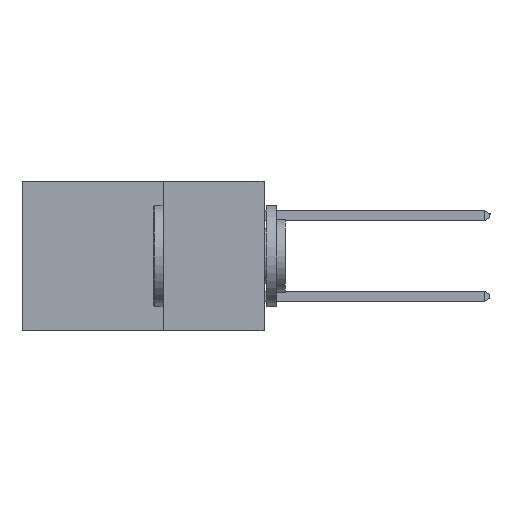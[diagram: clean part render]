
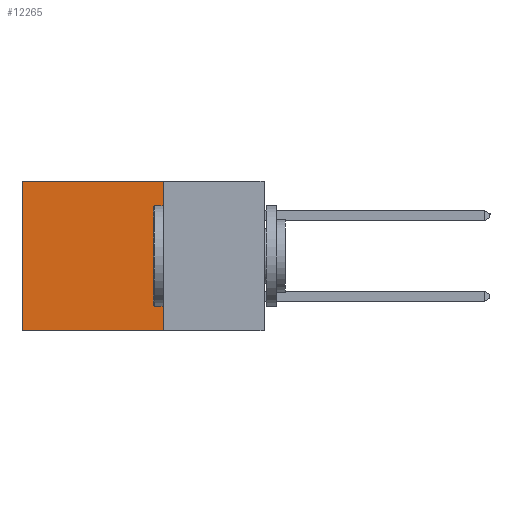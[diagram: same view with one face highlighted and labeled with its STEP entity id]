
A CAD part, left-side view. The second image highlights one B-rep face of the part: STEP entity #12265.
In plain terms, the highlighted planar face has unit normal (-1, 0, 0).
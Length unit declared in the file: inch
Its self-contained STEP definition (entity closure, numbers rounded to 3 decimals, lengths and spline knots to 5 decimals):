
#662 = DIRECTION ( 'NONE',  ( 1., 0., 0. ) ) ;
#748 = EDGE_CURVE ( 'NONE', #22641, #20299, #19825, .T. ) ;
#1297 = DIRECTION ( 'NONE',  ( 0., 1., 0. ) ) ;
#1557 = CARTESIAN_POINT ( 'NONE',  ( 0.2615, 0.25, 0. ) ) ;
#1861 = CARTESIAN_POINT ( 'NONE',  ( 0.2615, 0.25, -0.37 ) ) ;
#2840 = AXIS2_PLACEMENT_3D ( 'NONE', #23645, #662, #15559 ) ;
#3161 = VECTOR ( 'NONE', #1297, 39.37008 ) ;
#3678 = CARTESIAN_POINT ( 'NONE',  ( 0.2615, 0.25, -0.37 ) ) ;
#4022 = LINE ( 'NONE', #1861, #17274 ) ;
#4068 = VECTOR ( 'NONE', #26313, 39.37008 ) ;
#4404 = EDGE_LOOP ( 'NONE', ( #23438, #19910, #12541, #13023 ) ) ;
#4945 = LINE ( 'NONE', #16974, #21809 ) ;
#7323 = FACE_OUTER_BOUND ( 'NONE', #4404, .T. ) ;
#8329 = VERTEX_POINT ( 'NONE', #3678 ) ;
#10783 = CARTESIAN_POINT ( 'NONE',  ( 0.2615, 0.6, -0.37 ) ) ;
#12265 = ADVANCED_FACE ( 'NONE', ( #7323 ), #15156, .F. ) ;
#12541 = ORIENTED_EDGE ( 'NONE', *, *, #22267, .F. ) ;
#12747 = VERTEX_POINT ( 'NONE', #10783 ) ;
#13023 = ORIENTED_EDGE ( 'NONE', *, *, #748, .T. ) ;
#13257 = EDGE_CURVE ( 'NONE', #20299, #12747, #4945, .T. ) ;
#14011 = CARTESIAN_POINT ( 'NONE',  ( 0.2615, 0.25, -0.37 ) ) ;
#15156 = PLANE ( 'NONE',  #2840 ) ;
#15358 = DIRECTION ( 'NONE',  ( 0., 0., -1. ) ) ;
#15559 = DIRECTION ( 'NONE',  ( 0., 0., -1. ) ) ;
#16974 = CARTESIAN_POINT ( 'NONE',  ( 0.2615, 0.6, -0.37 ) ) ;
#17274 = VECTOR ( 'NONE', #24571, 39.37008 ) ;
#18073 = LINE ( 'NONE', #14011, #4068 ) ;
#18370 = CARTESIAN_POINT ( 'NONE',  ( 0.2615, 0.6, 0. ) ) ;
#18880 = EDGE_CURVE ( 'NONE', #8329, #12747, #4022, .T. ) ;
#19825 = LINE ( 'NONE', #1557, #3161 ) ;
#19910 = ORIENTED_EDGE ( 'NONE', *, *, #18880, .F. ) ;
#20299 = VERTEX_POINT ( 'NONE', #18370 ) ;
#21809 = VECTOR ( 'NONE', #15358, 39.37008 ) ;
#22267 = EDGE_CURVE ( 'NONE', #22641, #8329, #18073, .T. ) ;
#22641 = VERTEX_POINT ( 'NONE', #22975 ) ;
#22975 = CARTESIAN_POINT ( 'NONE',  ( 0.2615, 0.25, 0. ) ) ;
#23438 = ORIENTED_EDGE ( 'NONE', *, *, #13257, .T. ) ;
#23645 = CARTESIAN_POINT ( 'NONE',  ( 0.2615, 0.25, -0.37 ) ) ;
#24571 = DIRECTION ( 'NONE',  ( 0., 1., 0. ) ) ;
#26313 = DIRECTION ( 'NONE',  ( 0., 0., -1. ) ) ;
